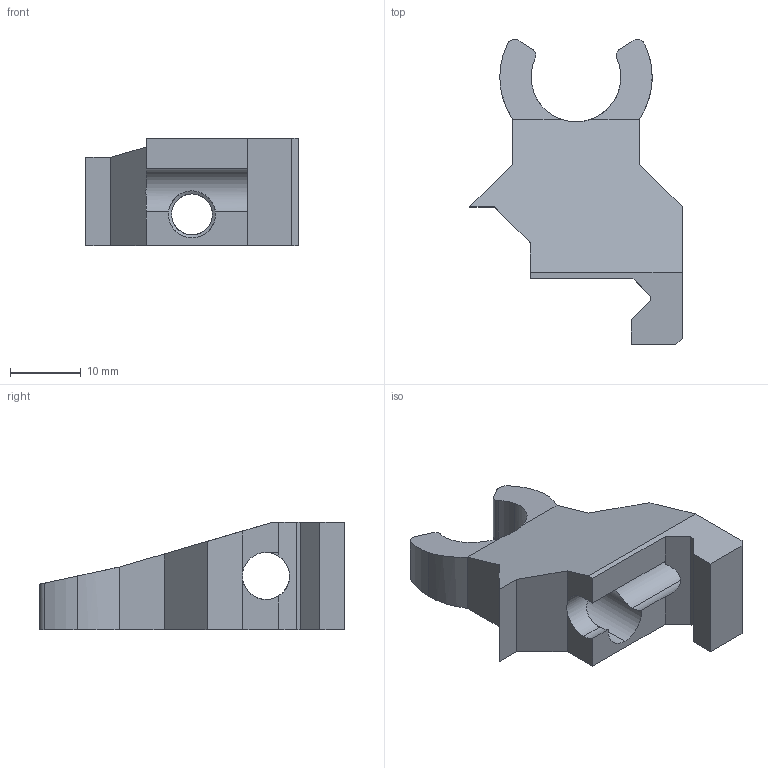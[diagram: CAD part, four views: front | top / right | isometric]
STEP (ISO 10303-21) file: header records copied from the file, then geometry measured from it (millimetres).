
FILE_DESCRIPTION (( 'STEP AP203' ), '1' );
FILE_NAME ('AF-WF-GS-PRT-001-STEP.STEP', '2020-07-21T19:01:20', ( '' ), ( '' ), 'SwSTEP 2.0', 'SolidWorks 2018', '' );
FILE_SCHEMA (( 'CONFIG_CONTROL_DESIGN' ));
Length unit declared in the file: inch
Products named in the file (1): AF-WF-GS-PRT-001-STEP
Bounding box: 30.1 x 43.23 x 15.24 mm (x, y, z)
Volume: 6222.6 mm3; surface area: 3742.9 mm2
Topology: 1 solids, 1 shells, 82 faces, 226 edges, 148 vertices
Faces by surface type: cylinder 41, plane 38, bspline 3
Entity records: 4192 total; most frequent: CARTESIAN_POINT 2196, ORIENTED_EDGE 452, DIRECTION 348, EDGE_CURVE 226, VERTEX_POINT 148, VECTOR 124, LINE 124, AXIS2_PLACEMENT_3D 112
